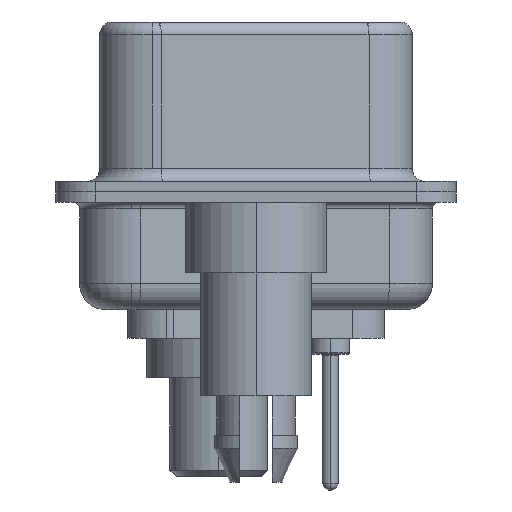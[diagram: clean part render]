
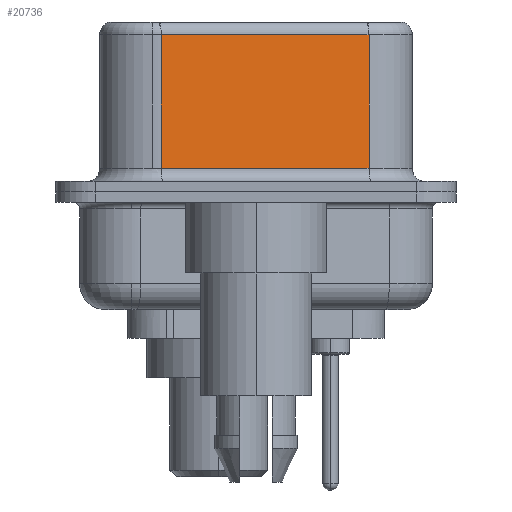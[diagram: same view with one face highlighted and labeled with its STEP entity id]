
A CAD part, left-side view. The second image highlights one B-rep face of the part: STEP entity #20736.
In plain terms, the highlighted planar face has unit normal (-0.985, -0.174, 0).
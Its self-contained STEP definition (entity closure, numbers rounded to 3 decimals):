
#642 = ORIENTED_EDGE ( 'NONE', *, *, #10579, .T. ) ;
#1049 = LINE ( 'NONE', #24767, #5870 ) ;
#1289 = VERTEX_POINT ( 'NONE', #23183 ) ;
#1751 = DIRECTION ( 'NONE',  ( -0.174, 0.985, 0. ) ) ;
#2452 = VERTEX_POINT ( 'NONE', #13520 ) ;
#2500 = VECTOR ( 'NONE', #1751, 1000. ) ;
#2632 = CARTESIAN_POINT ( 'NONE',  ( 5.132, -4.322, 0.9 ) ) ;
#2980 = VERTEX_POINT ( 'NONE', #18058 ) ;
#3070 = CARTESIAN_POINT ( 'NONE',  ( 3.73, 3.628, 6.52 ) ) ;
#4470 = LINE ( 'NONE', #21429, #10571 ) ;
#5136 = EDGE_CURVE ( 'NONE', #2452, #6793, #1049, .T. ) ;
#5870 = VECTOR ( 'NONE', #16094, 1000. ) ;
#6512 = FACE_OUTER_BOUND ( 'NONE', #15167, .T. ) ;
#6793 = VERTEX_POINT ( 'NONE', #2632 ) ;
#7293 = DIRECTION ( 'NONE',  ( 0.174, -0.985, 0. ) ) ;
#9362 = VECTOR ( 'NONE', #17301, 1000. ) ;
#10571 = VECTOR ( 'NONE', #7293, 1000. ) ;
#10579 = EDGE_CURVE ( 'NONE', #1289, #2980, #13464, .T. ) ;
#10693 = CARTESIAN_POINT ( 'NONE',  ( 5.132, -4.322, 6.52 ) ) ;
#10833 = AXIS2_PLACEMENT_3D ( 'NONE', #10693, #24799, #12730 ) ;
#12036 = ORIENTED_EDGE ( 'NONE', *, *, #12385, .T. ) ;
#12385 = EDGE_CURVE ( 'NONE', #2452, #1289, #18713, .T. ) ;
#12730 = DIRECTION ( 'NONE',  ( -0.174, 0.985, 0. ) ) ;
#13464 = LINE ( 'NONE', #3070, #9362 ) ;
#13520 = CARTESIAN_POINT ( 'NONE',  ( 5.132, -4.322, 6.02 ) ) ;
#15167 = EDGE_LOOP ( 'NONE', ( #24798, #12036, #642, #19391 ) ) ;
#16094 = DIRECTION ( 'NONE',  ( 0., 0., -1. ) ) ;
#16668 = PLANE ( 'NONE',  #10833 ) ;
#17301 = DIRECTION ( 'NONE',  ( 0., 0., -1. ) ) ;
#18058 = CARTESIAN_POINT ( 'NONE',  ( 3.73, 3.628, 0.9 ) ) ;
#18713 = LINE ( 'NONE', #26044, #2500 ) ;
#19391 = ORIENTED_EDGE ( 'NONE', *, *, #23058, .T. ) ;
#20736 = ADVANCED_FACE ( 'NONE', ( #6512 ), #16668, .F. ) ;
#21429 = CARTESIAN_POINT ( 'NONE',  ( 5.132, -4.322, 0.9 ) ) ;
#23058 = EDGE_CURVE ( 'NONE', #2980, #6793, #4470, .T. ) ;
#23183 = CARTESIAN_POINT ( 'NONE',  ( 3.73, 3.628, 6.02 ) ) ;
#24767 = CARTESIAN_POINT ( 'NONE',  ( 5.132, -4.322, 6.52 ) ) ;
#24798 = ORIENTED_EDGE ( 'NONE', *, *, #5136, .F. ) ;
#24799 = DIRECTION ( 'NONE',  ( 0.985, 0.174, 0. ) ) ;
#26044 = CARTESIAN_POINT ( 'NONE',  ( 5.132, -4.322, 6.02 ) ) ;
